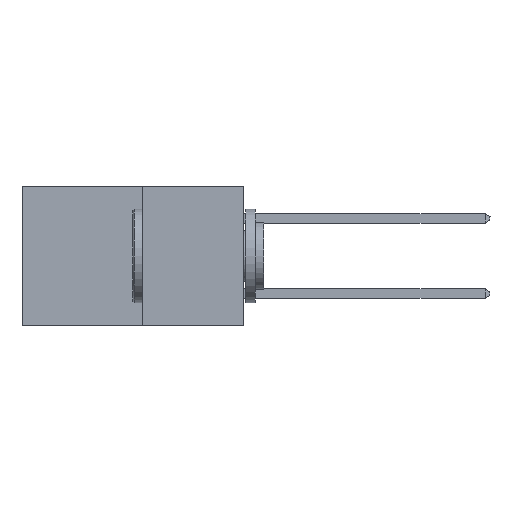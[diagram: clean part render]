
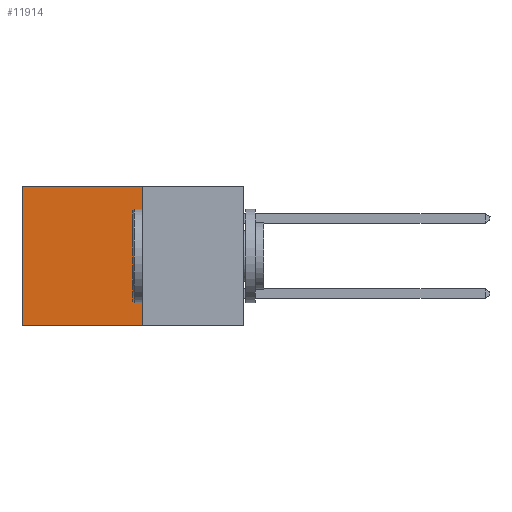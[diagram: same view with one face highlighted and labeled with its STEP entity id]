
A CAD part, left-side view. The second image highlights one B-rep face of the part: STEP entity #11914.
In plain terms, the highlighted planar face has unit normal (-1, 0, 0).
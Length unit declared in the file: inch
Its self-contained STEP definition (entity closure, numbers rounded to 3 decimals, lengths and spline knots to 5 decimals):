
#167 = FACE_OUTER_BOUND ( 'NONE', #10020, .T. ) ;
#208 = VERTEX_POINT ( 'NONE', #6463 ) ;
#850 = EDGE_CURVE ( 'NONE', #8391, #3071, #17994, .T. ) ;
#1442 = AXIS2_PLACEMENT_3D ( 'NONE', #16058, #16027, #15984 ) ;
#1555 = ORIENTED_EDGE ( 'NONE', *, *, #5717, .F. ) ;
#3071 = VERTEX_POINT ( 'NONE', #16489 ) ;
#3609 = VECTOR ( 'NONE', #4072, 39.37008 ) ;
#4013 = CARTESIAN_POINT ( 'NONE',  ( 0.277, 0.27, -0.37 ) ) ;
#4022 = LINE ( 'NONE', #11834, #6664 ) ;
#4072 = DIRECTION ( 'NONE',  ( 0., 0., -1. ) ) ;
#4139 = VERTEX_POINT ( 'NONE', #4013 ) ;
#4953 = ORIENTED_EDGE ( 'NONE', *, *, #8713, .T. ) ;
#5717 = EDGE_CURVE ( 'NONE', #8391, #4139, #4022, .T. ) ;
#6224 = ORIENTED_EDGE ( 'NONE', *, *, #11143, .F. ) ;
#6463 = CARTESIAN_POINT ( 'NONE',  ( 0.277, 0.59, -0.37 ) ) ;
#6664 = VECTOR ( 'NONE', #11741, 39.37008 ) ;
#7684 = CARTESIAN_POINT ( 'NONE',  ( 0.277, 0.27, 0. ) ) ;
#8180 = CARTESIAN_POINT ( 'NONE',  ( 0.277, 0.27, 0. ) ) ;
#8391 = VERTEX_POINT ( 'NONE', #7684 ) ;
#8713 = EDGE_CURVE ( 'NONE', #3071, #208, #15206, .T. ) ;
#9043 = LINE ( 'NONE', #12304, #16042 ) ;
#10020 = EDGE_LOOP ( 'NONE', ( #4953, #6224, #1555, #11647 ) ) ;
#10073 = CARTESIAN_POINT ( 'NONE',  ( 0.277, 0.59, -0.37 ) ) ;
#11143 = EDGE_CURVE ( 'NONE', #4139, #208, #9043, .T. ) ;
#11647 = ORIENTED_EDGE ( 'NONE', *, *, #850, .T. ) ;
#11741 = DIRECTION ( 'NONE',  ( 0., 0., -1. ) ) ;
#11834 = CARTESIAN_POINT ( 'NONE',  ( 0.277, 0.27, -0.37 ) ) ;
#11840 = DIRECTION ( 'NONE',  ( 0., 1., 0. ) ) ;
#11914 = ADVANCED_FACE ( 'NONE', ( #167 ), #17412, .F. ) ;
#12239 = DIRECTION ( 'NONE',  ( 0., 1., 0. ) ) ;
#12304 = CARTESIAN_POINT ( 'NONE',  ( 0.277, 0.27, -0.37 ) ) ;
#14169 = VECTOR ( 'NONE', #11840, 39.37008 ) ;
#15206 = LINE ( 'NONE', #10073, #3609 ) ;
#15984 = DIRECTION ( 'NONE',  ( 0., 0., -1. ) ) ;
#16027 = DIRECTION ( 'NONE',  ( 1., 0., 0. ) ) ;
#16042 = VECTOR ( 'NONE', #12239, 39.37008 ) ;
#16058 = CARTESIAN_POINT ( 'NONE',  ( 0.277, 0.27, -0.37 ) ) ;
#16489 = CARTESIAN_POINT ( 'NONE',  ( 0.277, 0.59, 0. ) ) ;
#17412 = PLANE ( 'NONE',  #1442 ) ;
#17994 = LINE ( 'NONE', #8180, #14169 ) ;
